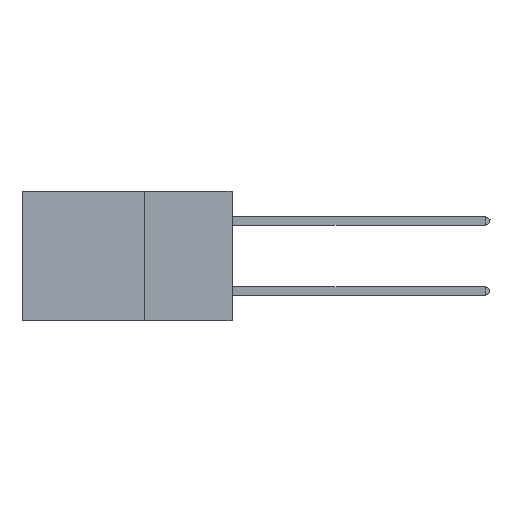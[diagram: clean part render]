
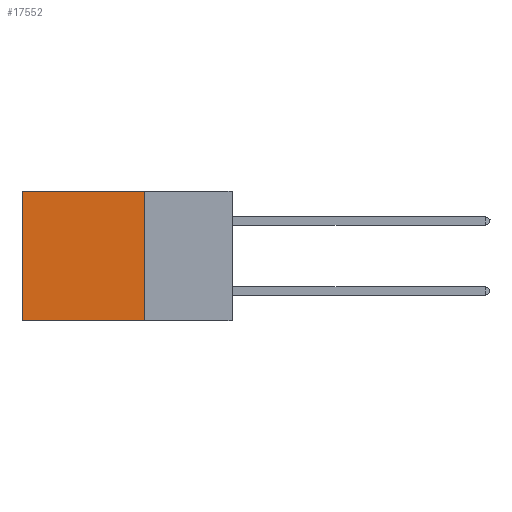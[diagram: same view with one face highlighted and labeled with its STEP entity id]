
A CAD part, left-side view. The second image highlights one B-rep face of the part: STEP entity #17552.
In plain terms, the highlighted planar face has unit normal (-1, 0, 0).
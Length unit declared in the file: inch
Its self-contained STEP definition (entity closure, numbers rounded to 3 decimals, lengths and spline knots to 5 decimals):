
#1803 = VECTOR ( 'NONE', #31370, 39.37008 ) ;
#2421 = VERTEX_POINT ( 'NONE', #25922 ) ;
#6358 = CARTESIAN_POINT ( 'NONE',  ( 0.2875, 0.6, 0. ) ) ;
#6704 = ORIENTED_EDGE ( 'NONE', *, *, #12108, .F. ) ;
#6795 = CARTESIAN_POINT ( 'NONE',  ( 0.2875, 0.6, -0.37 ) ) ;
#7100 = VECTOR ( 'NONE', #24170, 39.37008 ) ;
#7822 = VERTEX_POINT ( 'NONE', #27902 ) ;
#8008 = CARTESIAN_POINT ( 'NONE',  ( 0.2875, 0.25, 0. ) ) ;
#8673 = LINE ( 'NONE', #24000, #1803 ) ;
#11910 = ORIENTED_EDGE ( 'NONE', *, *, #23150, .T. ) ;
#12108 = EDGE_CURVE ( 'NONE', #7822, #2421, #8673, .T. ) ;
#15748 = PLANE ( 'NONE',  #16487 ) ;
#16487 = AXIS2_PLACEMENT_3D ( 'NONE', #8008, #26174, #18270 ) ;
#16614 = DIRECTION ( 'NONE',  ( 0., 0., -1. ) ) ;
#16725 = CARTESIAN_POINT ( 'NONE',  ( 0.2875, 0.6, 0. ) ) ;
#17204 = EDGE_CURVE ( 'NONE', #23110, #20562, #19474, .T. ) ;
#17552 = ADVANCED_FACE ( 'NONE', ( #24003 ), #15748, .F. ) ;
#17780 = VECTOR ( 'NONE', #25246, 39.37008 ) ;
#18270 = DIRECTION ( 'NONE',  ( 0., 0., -1. ) ) ;
#18939 = CARTESIAN_POINT ( 'NONE',  ( 0.2875, 0.25, 0. ) ) ;
#19474 = LINE ( 'NONE', #6358, #30970 ) ;
#20562 = VERTEX_POINT ( 'NONE', #6795 ) ;
#21474 = LINE ( 'NONE', #18939, #7100 ) ;
#22236 = EDGE_CURVE ( 'NONE', #2421, #20562, #22569, .T. ) ;
#22569 = LINE ( 'NONE', #32640, #17780 ) ;
#23110 = VERTEX_POINT ( 'NONE', #16725 ) ;
#23150 = EDGE_CURVE ( 'NONE', #7822, #23110, #21474, .T. ) ;
#23404 = EDGE_LOOP ( 'NONE', ( #27900, #26555, #6704, #11910 ) ) ;
#24000 = CARTESIAN_POINT ( 'NONE',  ( 0.2875, 0.25, 0. ) ) ;
#24003 = FACE_OUTER_BOUND ( 'NONE', #23404, .T. ) ;
#24170 = DIRECTION ( 'NONE',  ( 0., 1., 0. ) ) ;
#25246 = DIRECTION ( 'NONE',  ( 0., 1., 0. ) ) ;
#25922 = CARTESIAN_POINT ( 'NONE',  ( 0.2875, 0.25, -0.37 ) ) ;
#26174 = DIRECTION ( 'NONE',  ( 1., 0., 0. ) ) ;
#26555 = ORIENTED_EDGE ( 'NONE', *, *, #22236, .F. ) ;
#27900 = ORIENTED_EDGE ( 'NONE', *, *, #17204, .T. ) ;
#27902 = CARTESIAN_POINT ( 'NONE',  ( 0.2875, 0.25, 0. ) ) ;
#30970 = VECTOR ( 'NONE', #16614, 39.37008 ) ;
#31370 = DIRECTION ( 'NONE',  ( 0., 0., -1. ) ) ;
#32640 = CARTESIAN_POINT ( 'NONE',  ( 0.2875, 0.25, -0.37 ) ) ;
